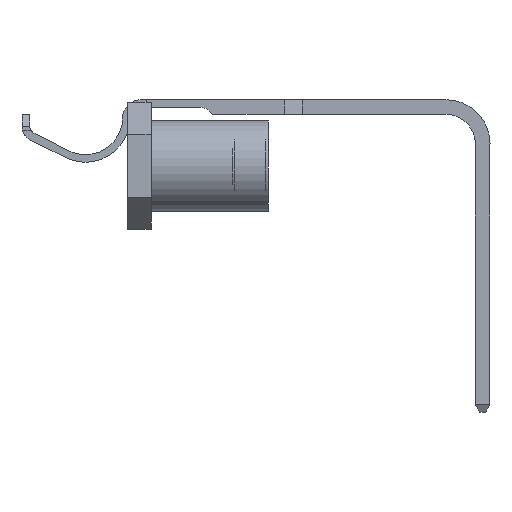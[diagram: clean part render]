
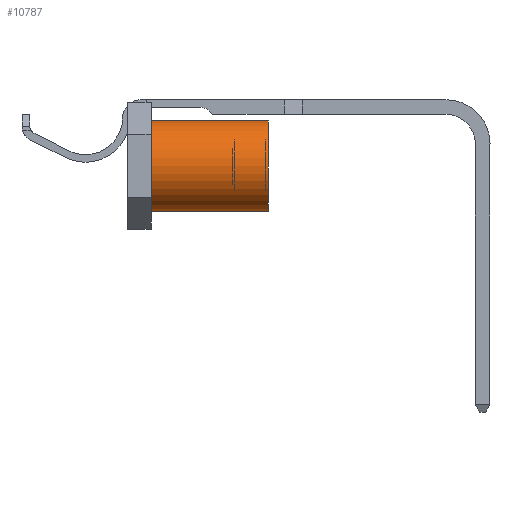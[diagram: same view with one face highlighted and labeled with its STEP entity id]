
A CAD part, left-side view. The second image highlights one B-rep face of the part: STEP entity #10787.
In plain terms, the highlighted cylindrical face has radius 1.968 mm (diameter 3.937 mm), a partial arc.
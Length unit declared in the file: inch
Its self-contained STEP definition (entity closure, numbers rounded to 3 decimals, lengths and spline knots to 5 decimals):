
#1418 = CARTESIAN_POINT ( 'NONE',  ( 0., 0.24, -0.0775 ) ) ;
#1438 = EDGE_CURVE ( 'NONE', #24370, #15530, #8549, .T. ) ;
#3766 = VECTOR ( 'NONE', #13344, 39.37008 ) ;
#3962 = DIRECTION ( 'NONE',  ( 0., -1., 0. ) ) ;
#5105 = CIRCLE ( 'NONE', #24692, 0.0775 ) ;
#6617 = FACE_OUTER_BOUND ( 'NONE', #16451, .T. ) ;
#7137 = DIRECTION ( 'NONE',  ( 0., 1., 0. ) ) ;
#8549 = LINE ( 'NONE', #1418, #14435 ) ;
#8912 = EDGE_CURVE ( 'NONE', #24370, #9496, #5105, .T. ) ;
#9496 = VERTEX_POINT ( 'NONE', #12436 ) ;
#10311 = CARTESIAN_POINT ( 'NONE',  ( 0., 0.04, 0.0775 ) ) ;
#10787 = ADVANCED_FACE ( 'NONE', ( #6617 ), #25694, .T. ) ;
#10979 = ORIENTED_EDGE ( 'NONE', *, *, #1438, .T. ) ;
#11631 = ORIENTED_EDGE ( 'NONE', *, *, #8912, .F. ) ;
#12436 = CARTESIAN_POINT ( 'NONE',  ( 0., 0.24, 0.0775 ) ) ;
#12573 = CARTESIAN_POINT ( 'NONE',  ( 0., 0.24, 0. ) ) ;
#12662 = CARTESIAN_POINT ( 'NONE',  ( 0., 0.24, 0. ) ) ;
#12689 = ORIENTED_EDGE ( 'NONE', *, *, #16559, .T. ) ;
#13344 = DIRECTION ( 'NONE',  ( 0., -1., 0. ) ) ;
#14379 = AXIS2_PLACEMENT_3D ( 'NONE', #12573, #19830, #29895 ) ;
#14435 = VECTOR ( 'NONE', #3962, 39.37008 ) ;
#15134 = DIRECTION ( 'NONE',  ( 0., 0., 1. ) ) ;
#15530 = VERTEX_POINT ( 'NONE', #22927 ) ;
#15557 = ORIENTED_EDGE ( 'NONE', *, *, #28003, .F. ) ;
#16451 = EDGE_LOOP ( 'NONE', ( #15557, #11631, #10979, #12689 ) ) ;
#16559 = EDGE_CURVE ( 'NONE', #15530, #18898, #29652, .T. ) ;
#18898 = VERTEX_POINT ( 'NONE', #10311 ) ;
#19830 = DIRECTION ( 'NONE',  ( 0., -1., 0. ) ) ;
#20819 = AXIS2_PLACEMENT_3D ( 'NONE', #21988, #7137, #24519 ) ;
#21988 = CARTESIAN_POINT ( 'NONE',  ( 0., 0.04, 0. ) ) ;
#22927 = CARTESIAN_POINT ( 'NONE',  ( 0., 0.04, -0.0775 ) ) ;
#24370 = VERTEX_POINT ( 'NONE', #26416 ) ;
#24519 = DIRECTION ( 'NONE',  ( 0., 0., 1. ) ) ;
#24692 = AXIS2_PLACEMENT_3D ( 'NONE', #12662, #29989, #15134 ) ;
#25667 = CARTESIAN_POINT ( 'NONE',  ( 0., 0.24, 0.0775 ) ) ;
#25694 = CYLINDRICAL_SURFACE ( 'NONE', #14379, 0.0775 ) ;
#26416 = CARTESIAN_POINT ( 'NONE',  ( 0., 0.24, -0.0775 ) ) ;
#28003 = EDGE_CURVE ( 'NONE', #9496, #18898, #30327, .T. ) ;
#29652 = CIRCLE ( 'NONE', #20819, 0.0775 ) ;
#29895 = DIRECTION ( 'NONE',  ( 0., 0., -1. ) ) ;
#29989 = DIRECTION ( 'NONE',  ( 0., 1., 0. ) ) ;
#30327 = LINE ( 'NONE', #25667, #3766 ) ;
